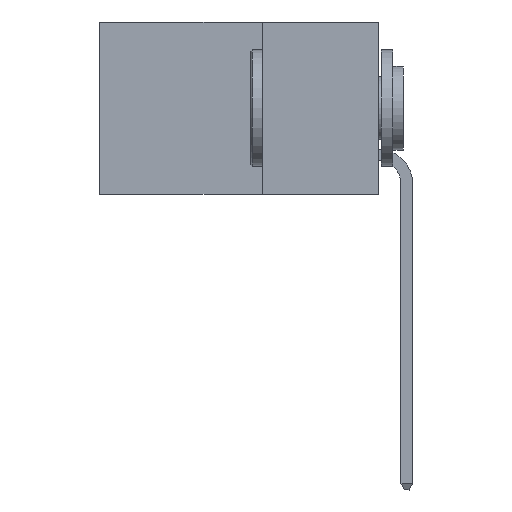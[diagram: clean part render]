
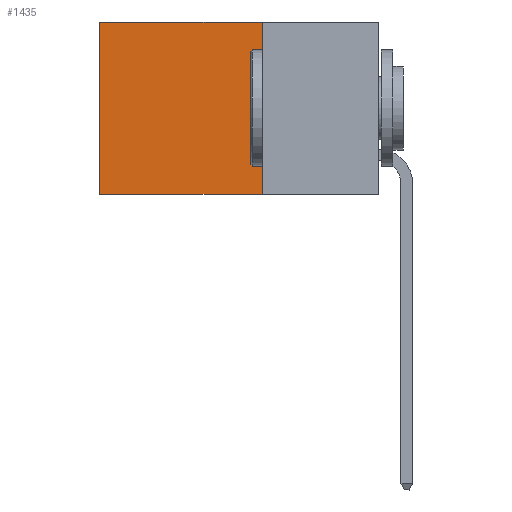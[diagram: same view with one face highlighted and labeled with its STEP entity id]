
A CAD part, left-side view. The second image highlights one B-rep face of the part: STEP entity #1435.
In plain terms, the highlighted planar face has unit normal (-1, 0, 0).
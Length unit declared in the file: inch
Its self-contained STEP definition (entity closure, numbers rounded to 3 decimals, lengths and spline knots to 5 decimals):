
#44 = CARTESIAN_POINT ( 'NONE',  ( 0.298, 0.25, 0. ) ) ;
#188 = ORIENTED_EDGE ( 'NONE', *, *, #3376, .F. ) ;
#464 = AXIS2_PLACEMENT_3D ( 'NONE', #44, #1729, #1845 ) ;
#1326 = CARTESIAN_POINT ( 'NONE',  ( 0.298, 0.25, -0.37 ) ) ;
#1435 = ADVANCED_FACE ( 'NONE', ( #10500 ), #6273, .F. ) ;
#1729 = DIRECTION ( 'NONE',  ( 1., 0., 0. ) ) ;
#1845 = DIRECTION ( 'NONE',  ( 0., 0., -1. ) ) ;
#2181 = ORIENTED_EDGE ( 'NONE', *, *, #13810, .T. ) ;
#2541 = CARTESIAN_POINT ( 'NONE',  ( 0.298, 0.25, -0.37 ) ) ;
#3376 = EDGE_CURVE ( 'NONE', #20011, #5844, #25421, .T. ) ;
#3924 = EDGE_CURVE ( 'NONE', #20011, #8780, #6805, .T. ) ;
#4225 = VECTOR ( 'NONE', #24436, 39.37008 ) ;
#5750 = ORIENTED_EDGE ( 'NONE', *, *, #10356, .F. ) ;
#5844 = VERTEX_POINT ( 'NONE', #1326 ) ;
#6273 = PLANE ( 'NONE',  #464 ) ;
#6412 = CARTESIAN_POINT ( 'NONE',  ( 0.298, 0.6, -0.37 ) ) ;
#6805 = LINE ( 'NONE', #20420, #16751 ) ;
#8780 = VERTEX_POINT ( 'NONE', #21907 ) ;
#9550 = LINE ( 'NONE', #2541, #14823 ) ;
#10305 = CARTESIAN_POINT ( 'NONE',  ( 0.298, 0.25, 0. ) ) ;
#10356 = EDGE_CURVE ( 'NONE', #5844, #12934, #9550, .T. ) ;
#10500 = FACE_OUTER_BOUND ( 'NONE', #21210, .T. ) ;
#12934 = VERTEX_POINT ( 'NONE', #6412 ) ;
#12951 = CARTESIAN_POINT ( 'NONE',  ( 0.298, 0.6, 0. ) ) ;
#13617 = ORIENTED_EDGE ( 'NONE', *, *, #3924, .T. ) ;
#13810 = EDGE_CURVE ( 'NONE', #8780, #12934, #25678, .T. ) ;
#14823 = VECTOR ( 'NONE', #16427, 39.37008 ) ;
#16427 = DIRECTION ( 'NONE',  ( 0., 1., 0. ) ) ;
#16751 = VECTOR ( 'NONE', #20519, 39.37008 ) ;
#19020 = DIRECTION ( 'NONE',  ( 0., 0., -1. ) ) ;
#19095 = VECTOR ( 'NONE', #19020, 39.37008 ) ;
#20011 = VERTEX_POINT ( 'NONE', #10305 ) ;
#20420 = CARTESIAN_POINT ( 'NONE',  ( 0.298, 0.25, 0. ) ) ;
#20519 = DIRECTION ( 'NONE',  ( 0., 1., 0. ) ) ;
#21210 = EDGE_LOOP ( 'NONE', ( #2181, #5750, #188, #13617 ) ) ;
#21907 = CARTESIAN_POINT ( 'NONE',  ( 0.298, 0.6, 0. ) ) ;
#23036 = CARTESIAN_POINT ( 'NONE',  ( 0.298, 0.25, 0. ) ) ;
#24436 = DIRECTION ( 'NONE',  ( 0., 0., -1. ) ) ;
#25421 = LINE ( 'NONE', #23036, #4225 ) ;
#25678 = LINE ( 'NONE', #12951, #19095 ) ;
